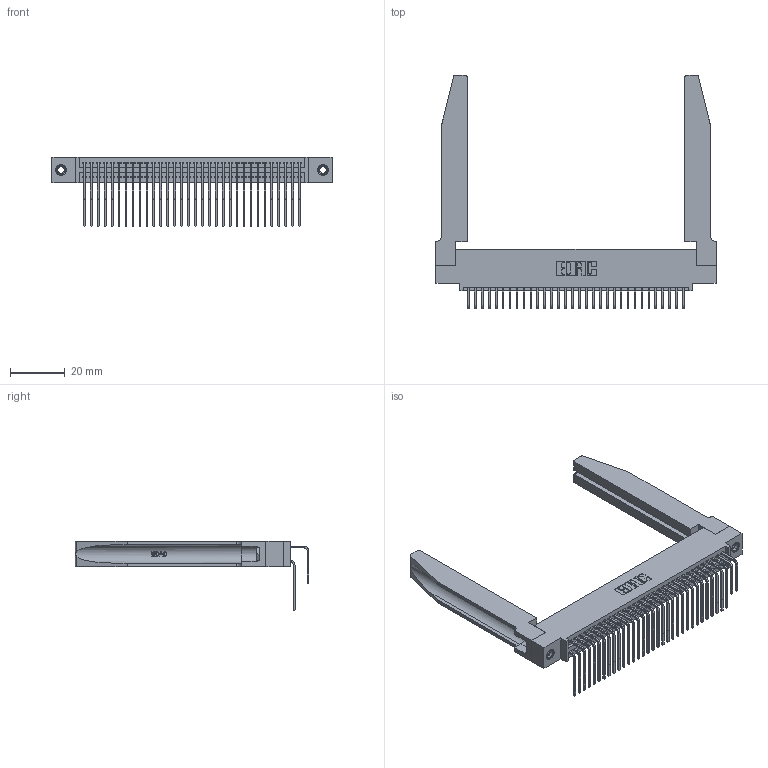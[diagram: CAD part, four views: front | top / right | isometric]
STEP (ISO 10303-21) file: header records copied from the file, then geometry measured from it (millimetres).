
FILE_DESCRIPTION (( 'STEP AP203' ), '1' );
FILE_NAME ('345-064-558-578.STEP', '2019-10-30T15:15:56', ( '' ), ( '' ), 'SwSTEP 2.0', 'SolidWorks 2016', '' );
FILE_SCHEMA (( 'CONFIG_CONTROL_DESIGN' ));
Length unit declared in the file: inch
Products named in the file (6): 345-250-001_345-250-001-102; 345-064-558-578; 345-220-078_345-220-078; 345 Part_0.110 Offset - 0.156 Dia-TH; 345-292-001_558 Tail - 2; 345-292-001_558 559 Tail - 1
Assembly tree (69 placements, depth 2):
  345-064-558-578
    345 Part_0.110 Offset - 0.156 Dia-TH
    345-292-001_558 559 Tail - 1  x32
    345-292-001_558 Tail - 2  x32
    345-250-001_345-250-001-102  x2
    345-220-078_345-220-078  x2
Bounding box: 102.51 x 85.59 x 25.53 mm (x, y, z)
Volume: 17931.8 mm3; surface area: 23493.9 mm2
Topology: 69 solids, 69 shells, 3692 faces, 10881 edges, 7158 vertices
Faces by surface type: plane 2466, cylinder 1174, bspline 36, cone 12, torus 4
Entity records: 32978 total; most frequent: CARTESIAN_POINT 6502, ORIENTED_EDGE 5282, DIRECTION 4711, EDGE_CURVE 2641, VECTOR 2247, LINE 2247, VERTEX_POINT 1752, AXIS2_PLACEMENT_3D 1232
